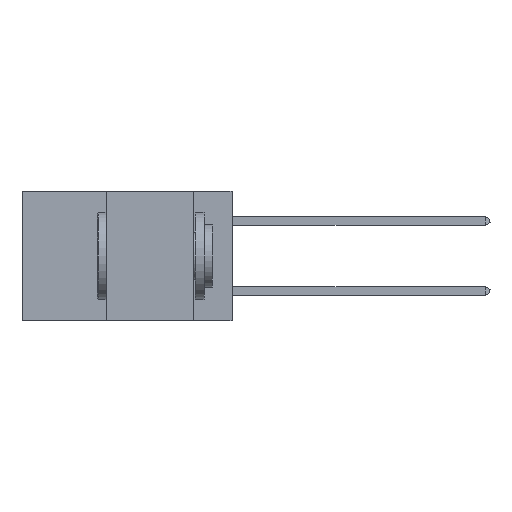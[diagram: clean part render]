
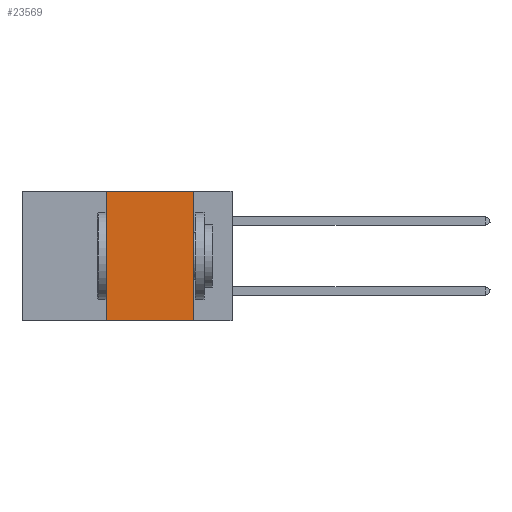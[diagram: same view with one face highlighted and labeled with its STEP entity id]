
A CAD part, left-side view. The second image highlights one B-rep face of the part: STEP entity #23569.
In plain terms, the highlighted planar face has unit normal (-1, 0, 0).
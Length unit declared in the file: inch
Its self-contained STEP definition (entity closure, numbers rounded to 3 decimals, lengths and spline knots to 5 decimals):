
#146 = CARTESIAN_POINT ( 'NONE',  ( 0., 0.11, 0. ) ) ;
#406 = CARTESIAN_POINT ( 'NONE',  ( 0., 0.36, 0. ) ) ;
#1033 = LINE ( 'NONE', #10785, #24060 ) ;
#3211 = DIRECTION ( 'NONE',  ( 0., -1., 0. ) ) ;
#3249 = ORIENTED_EDGE ( 'NONE', *, *, #7277, .F. ) ;
#4225 = VERTEX_POINT ( 'NONE', #26676 ) ;
#4315 = EDGE_CURVE ( 'NONE', #32899, #4225, #15283, .T. ) ;
#4448 = CARTESIAN_POINT ( 'NONE',  ( 0., 0.11, -0.37 ) ) ;
#5193 = VECTOR ( 'NONE', #3211, 39.37008 ) ;
#7277 = EDGE_CURVE ( 'NONE', #8649, #32062, #1033, .T. ) ;
#8649 = VERTEX_POINT ( 'NONE', #146 ) ;
#9005 = LINE ( 'NONE', #9377, #5193 ) ;
#9377 = CARTESIAN_POINT ( 'NONE',  ( 0., 0.6, -0.37 ) ) ;
#10392 = EDGE_LOOP ( 'NONE', ( #3249, #24762, #20121, #31041 ) ) ;
#10785 = CARTESIAN_POINT ( 'NONE',  ( 0., 0.11, 0. ) ) ;
#14240 = PLANE ( 'NONE',  #28988 ) ;
#15283 = LINE ( 'NONE', #406, #26555 ) ;
#15649 = DIRECTION ( 'NONE',  ( 0., 0., 1. ) ) ;
#17228 = VECTOR ( 'NONE', #20812, 39.37008 ) ;
#18405 = FACE_OUTER_BOUND ( 'NONE', #10392, .T. ) ;
#19648 = CARTESIAN_POINT ( 'NONE',  ( 0., 0.6, 0. ) ) ;
#20121 = ORIENTED_EDGE ( 'NONE', *, *, #4315, .F. ) ;
#20286 = CARTESIAN_POINT ( 'NONE',  ( 0., 0.6, 0. ) ) ;
#20526 = EDGE_CURVE ( 'NONE', #4225, #8649, #23830, .T. ) ;
#20812 = DIRECTION ( 'NONE',  ( 0., -1., 0. ) ) ;
#23270 = DIRECTION ( 'NONE',  ( 0., 0., -1. ) ) ;
#23569 = ADVANCED_FACE ( 'NONE', ( #18405 ), #14240, .F. ) ;
#23830 = LINE ( 'NONE', #20286, #17228 ) ;
#24060 = VECTOR ( 'NONE', #23270, 39.37008 ) ;
#24762 = ORIENTED_EDGE ( 'NONE', *, *, #20526, .F. ) ;
#25920 = CARTESIAN_POINT ( 'NONE',  ( 0., 0.36, -0.37 ) ) ;
#26555 = VECTOR ( 'NONE', #15649, 39.37008 ) ;
#26676 = CARTESIAN_POINT ( 'NONE',  ( 0., 0.36, 0. ) ) ;
#28988 = AXIS2_PLACEMENT_3D ( 'NONE', #19648, #35072, #29095 ) ;
#29095 = DIRECTION ( 'NONE',  ( 0., 0., -1. ) ) ;
#31041 = ORIENTED_EDGE ( 'NONE', *, *, #36505, .T. ) ;
#32062 = VERTEX_POINT ( 'NONE', #4448 ) ;
#32899 = VERTEX_POINT ( 'NONE', #25920 ) ;
#35072 = DIRECTION ( 'NONE',  ( 1., 0., 0. ) ) ;
#36505 = EDGE_CURVE ( 'NONE', #32899, #32062, #9005, .T. ) ;
